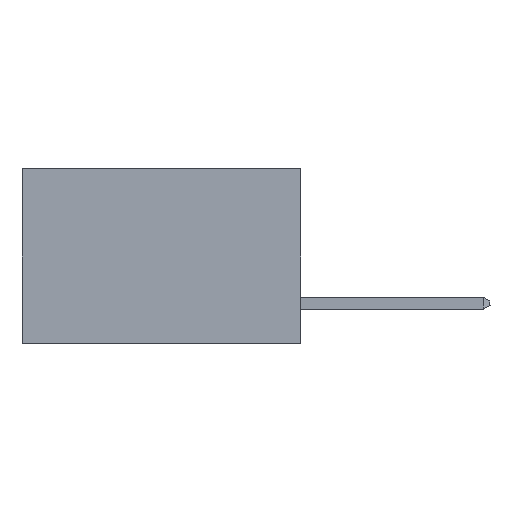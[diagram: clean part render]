
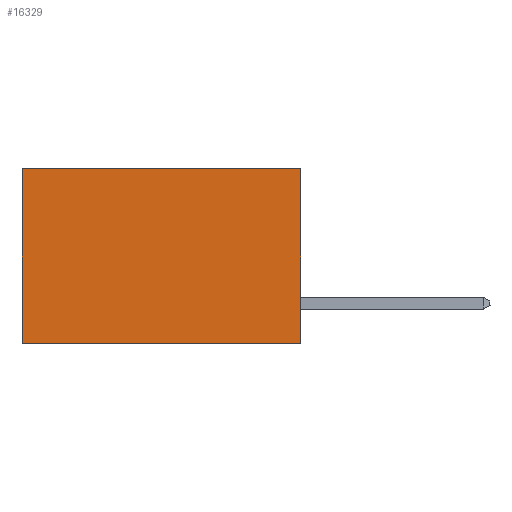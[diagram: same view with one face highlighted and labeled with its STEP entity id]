
A CAD part, left-side view. The second image highlights one B-rep face of the part: STEP entity #16329.
In plain terms, the highlighted planar face has unit normal (-1, 0, 0).
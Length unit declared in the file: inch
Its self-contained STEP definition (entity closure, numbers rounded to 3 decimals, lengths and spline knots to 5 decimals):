
#586 = DIRECTION ( 'NONE',  ( 0., 1., 0. ) ) ;
#1226 = PLANE ( 'NONE',  #4344 ) ;
#1494 = DIRECTION ( 'NONE',  ( 0., 0., -1. ) ) ;
#2287 = ORIENTED_EDGE ( 'NONE', *, *, #19545, .F. ) ;
#2764 = ORIENTED_EDGE ( 'NONE', *, *, #7130, .F. ) ;
#4344 = AXIS2_PLACEMENT_3D ( 'NONE', #17520, #5383, #19768 ) ;
#5031 = DIRECTION ( 'NONE',  ( 0., 1., 0. ) ) ;
#5383 = DIRECTION ( 'NONE',  ( 1., 0., 0. ) ) ;
#5397 = VERTEX_POINT ( 'NONE', #23009 ) ;
#5518 = CARTESIAN_POINT ( 'NONE',  ( 0.277, 0., -0.37 ) ) ;
#6228 = CARTESIAN_POINT ( 'NONE',  ( 0.277, 0., -0.37 ) ) ;
#7130 = EDGE_CURVE ( 'NONE', #7493, #8593, #24437, .T. ) ;
#7493 = VERTEX_POINT ( 'NONE', #11209 ) ;
#8593 = VERTEX_POINT ( 'NONE', #9819 ) ;
#9819 = CARTESIAN_POINT ( 'NONE',  ( 0.277, 0.59, -0.37 ) ) ;
#10873 = CARTESIAN_POINT ( 'NONE',  ( 0.277, 0.59, 0. ) ) ;
#11209 = CARTESIAN_POINT ( 'NONE',  ( 0.277, 0., -0.37 ) ) ;
#11680 = LINE ( 'NONE', #12921, #16507 ) ;
#12249 = LINE ( 'NONE', #6228, #13525 ) ;
#12921 = CARTESIAN_POINT ( 'NONE',  ( 0.277, 0., 0. ) ) ;
#13138 = LINE ( 'NONE', #22082, #23540 ) ;
#13291 = VERTEX_POINT ( 'NONE', #10873 ) ;
#13525 = VECTOR ( 'NONE', #20646, 39.37008 ) ;
#16329 = ADVANCED_FACE ( 'NONE', ( #18660 ), #1226, .F. ) ;
#16507 = VECTOR ( 'NONE', #586, 39.37008 ) ;
#17520 = CARTESIAN_POINT ( 'NONE',  ( 0.277, 0., -0.37 ) ) ;
#17574 = VECTOR ( 'NONE', #5031, 39.37008 ) ;
#18378 = EDGE_CURVE ( 'NONE', #5397, #13291, #11680, .T. ) ;
#18660 = FACE_OUTER_BOUND ( 'NONE', #26666, .T. ) ;
#19545 = EDGE_CURVE ( 'NONE', #5397, #7493, #12249, .T. ) ;
#19768 = DIRECTION ( 'NONE',  ( 0., 0., -1. ) ) ;
#20090 = ORIENTED_EDGE ( 'NONE', *, *, #21305, .T. ) ;
#20646 = DIRECTION ( 'NONE',  ( 0., 0., -1. ) ) ;
#20916 = ORIENTED_EDGE ( 'NONE', *, *, #18378, .T. ) ;
#21305 = EDGE_CURVE ( 'NONE', #13291, #8593, #13138, .T. ) ;
#22082 = CARTESIAN_POINT ( 'NONE',  ( 0.277, 0.59, -0.37 ) ) ;
#23009 = CARTESIAN_POINT ( 'NONE',  ( 0.277, 0., 0. ) ) ;
#23540 = VECTOR ( 'NONE', #1494, 39.37008 ) ;
#24437 = LINE ( 'NONE', #5518, #17574 ) ;
#26666 = EDGE_LOOP ( 'NONE', ( #20090, #2764, #2287, #20916 ) ) ;
